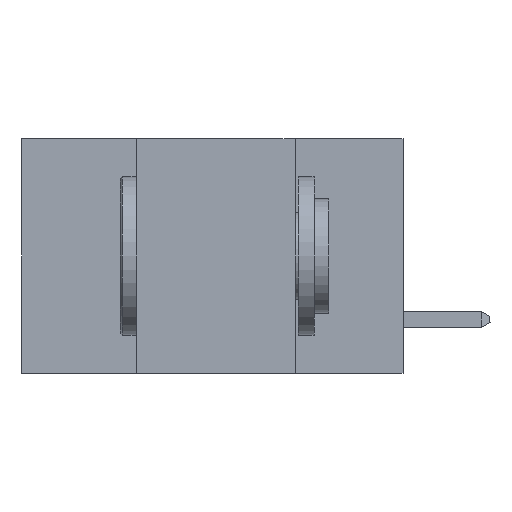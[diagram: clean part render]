
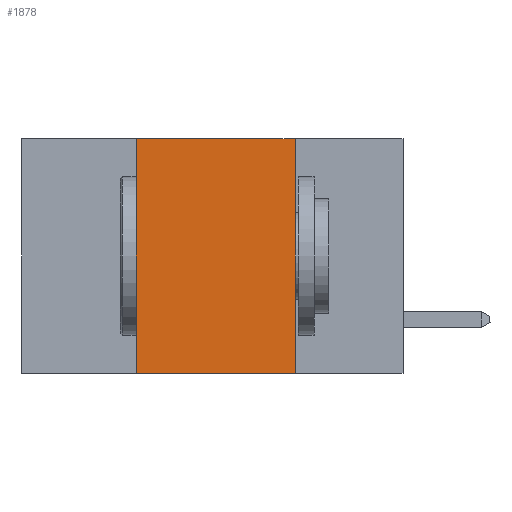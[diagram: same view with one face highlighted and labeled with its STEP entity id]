
A CAD part, left-side view. The second image highlights one B-rep face of the part: STEP entity #1878.
In plain terms, the highlighted planar face has unit normal (-1, 0, 0).
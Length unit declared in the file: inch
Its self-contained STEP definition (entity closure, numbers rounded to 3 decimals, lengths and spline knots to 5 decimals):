
#1878 = ADVANCED_FACE ( 'NONE', ( #2474 ), #6936, .F. ) ;
#2474 = FACE_OUTER_BOUND ( 'NONE', #9314, .T. ) ;
#2669 = VECTOR ( 'NONE', #22822, 39.37008 ) ;
#2720 = LINE ( 'NONE', #19323, #3362 ) ;
#2916 = LINE ( 'NONE', #3499, #25747 ) ;
#2920 = ORIENTED_EDGE ( 'NONE', *, *, #23395, .F. ) ;
#3362 = VECTOR ( 'NONE', #13022, 39.37008 ) ;
#3499 = CARTESIAN_POINT ( 'NONE',  ( 0., 0.6, -0.37 ) ) ;
#5086 = CARTESIAN_POINT ( 'NONE',  ( 0., 0.17, 0. ) ) ;
#5474 = VECTOR ( 'NONE', #11677, 39.37008 ) ;
#6742 = ORIENTED_EDGE ( 'NONE', *, *, #24372, .F. ) ;
#6936 = PLANE ( 'NONE',  #13033 ) ;
#7355 = ORIENTED_EDGE ( 'NONE', *, *, #12750, .T. ) ;
#7607 = VERTEX_POINT ( 'NONE', #10848 ) ;
#9314 = EDGE_LOOP ( 'NONE', ( #10533, #2920, #6742, #7355 ) ) ;
#10501 = DIRECTION ( 'NONE',  ( 0., -1., 0. ) ) ;
#10533 = ORIENTED_EDGE ( 'NONE', *, *, #14317, .F. ) ;
#10606 = LINE ( 'NONE', #18413, #2669 ) ;
#10848 = CARTESIAN_POINT ( 'NONE',  ( 0., 0.42, -0.37 ) ) ;
#11459 = LINE ( 'NONE', #17464, #5474 ) ;
#11677 = DIRECTION ( 'NONE',  ( 0., 0., -1. ) ) ;
#12750 = EDGE_CURVE ( 'NONE', #7607, #19002, #2916, .T. ) ;
#13022 = DIRECTION ( 'NONE',  ( 0., -1., 0. ) ) ;
#13033 = AXIS2_PLACEMENT_3D ( 'NONE', #19414, #19231, #19068 ) ;
#14317 = EDGE_CURVE ( 'NONE', #15378, #19002, #11459, .T. ) ;
#15378 = VERTEX_POINT ( 'NONE', #5086 ) ;
#17464 = CARTESIAN_POINT ( 'NONE',  ( 0., 0.17, 0. ) ) ;
#18413 = CARTESIAN_POINT ( 'NONE',  ( 0., 0.42, 0. ) ) ;
#19002 = VERTEX_POINT ( 'NONE', #26021 ) ;
#19068 = DIRECTION ( 'NONE',  ( 0., 0., -1. ) ) ;
#19148 = VERTEX_POINT ( 'NONE', #22155 ) ;
#19231 = DIRECTION ( 'NONE',  ( 1., 0., 0. ) ) ;
#19323 = CARTESIAN_POINT ( 'NONE',  ( 0., 0.6, 0. ) ) ;
#19414 = CARTESIAN_POINT ( 'NONE',  ( 0., 0.6, 0. ) ) ;
#22155 = CARTESIAN_POINT ( 'NONE',  ( 0., 0.42, 0. ) ) ;
#22822 = DIRECTION ( 'NONE',  ( 0., 0., 1. ) ) ;
#23395 = EDGE_CURVE ( 'NONE', #19148, #15378, #2720, .T. ) ;
#24372 = EDGE_CURVE ( 'NONE', #7607, #19148, #10606, .T. ) ;
#25747 = VECTOR ( 'NONE', #10501, 39.37008 ) ;
#26021 = CARTESIAN_POINT ( 'NONE',  ( 0., 0.17, -0.37 ) ) ;
